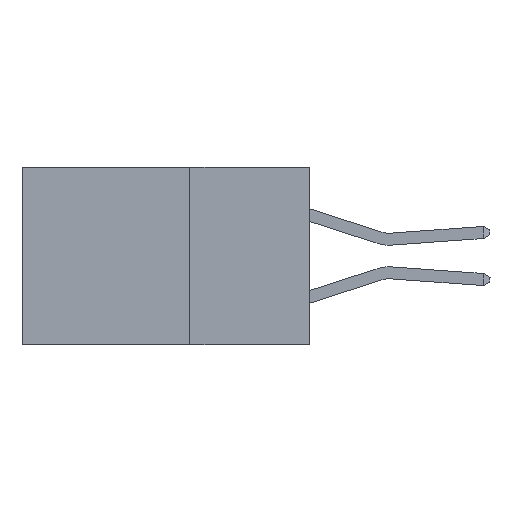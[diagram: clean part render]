
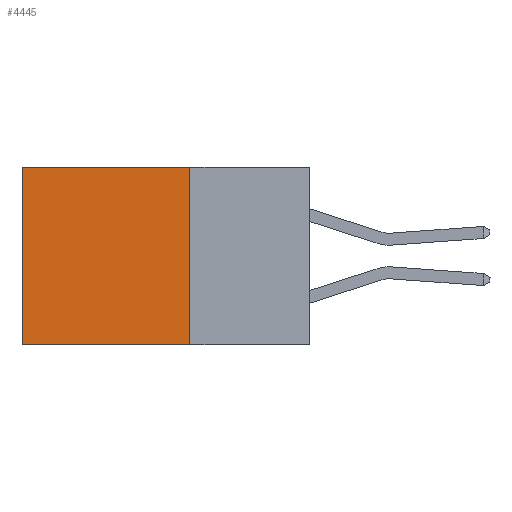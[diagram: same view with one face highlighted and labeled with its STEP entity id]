
A CAD part, left-side view. The second image highlights one B-rep face of the part: STEP entity #4445.
In plain terms, the highlighted planar face has unit normal (-1, 0, 0).
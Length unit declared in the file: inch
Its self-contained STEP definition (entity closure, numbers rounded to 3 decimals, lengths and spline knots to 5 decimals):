
#317 = EDGE_CURVE ( 'NONE', #3598, #5540, #5479, .T. ) ;
#974 = ORIENTED_EDGE ( 'NONE', *, *, #4265, .F. ) ;
#1936 = DIRECTION ( 'NONE',  ( 0., 0., -1. ) ) ;
#2107 = VECTOR ( 'NONE', #5605, 39.37008 ) ;
#2626 = EDGE_LOOP ( 'NONE', ( #6995, #974, #3247, #8632 ) ) ;
#2627 = LINE ( 'NONE', #6572, #8581 ) ;
#2744 = EDGE_CURVE ( 'NONE', #3598, #6791, #6237, .T. ) ;
#2918 = CARTESIAN_POINT ( 'NONE',  ( 0.298, 0.25, -0.37 ) ) ;
#3144 = LINE ( 'NONE', #2918, #8501 ) ;
#3247 = ORIENTED_EDGE ( 'NONE', *, *, #317, .F. ) ;
#3266 = CARTESIAN_POINT ( 'NONE',  ( 0.298, 0.6, 0. ) ) ;
#3598 = VERTEX_POINT ( 'NONE', #4420 ) ;
#3642 = FACE_OUTER_BOUND ( 'NONE', #2626, .T. ) ;
#3673 = DIRECTION ( 'NONE',  ( 0., 1., 0. ) ) ;
#4136 = CARTESIAN_POINT ( 'NONE',  ( 0.298, 0.25, 0. ) ) ;
#4265 = EDGE_CURVE ( 'NONE', #5540, #5332, #3144, .T. ) ;
#4420 = CARTESIAN_POINT ( 'NONE',  ( 0.298, 0.25, 0. ) ) ;
#4445 = ADVANCED_FACE ( 'NONE', ( #3642 ), #5028, .F. ) ;
#5028 = PLANE ( 'NONE',  #7657 ) ;
#5332 = VERTEX_POINT ( 'NONE', #6177 ) ;
#5479 = LINE ( 'NONE', #9676, #9493 ) ;
#5540 = VERTEX_POINT ( 'NONE', #6692 ) ;
#5605 = DIRECTION ( 'NONE',  ( 0., 1., 0. ) ) ;
#6177 = CARTESIAN_POINT ( 'NONE',  ( 0.298, 0.6, -0.37 ) ) ;
#6237 = LINE ( 'NONE', #9410, #2107 ) ;
#6572 = CARTESIAN_POINT ( 'NONE',  ( 0.298, 0.6, 0. ) ) ;
#6657 = EDGE_CURVE ( 'NONE', #6791, #5332, #2627, .T. ) ;
#6679 = DIRECTION ( 'NONE',  ( 0., 0., -1. ) ) ;
#6692 = CARTESIAN_POINT ( 'NONE',  ( 0.298, 0.25, -0.37 ) ) ;
#6791 = VERTEX_POINT ( 'NONE', #3266 ) ;
#6995 = ORIENTED_EDGE ( 'NONE', *, *, #6657, .T. ) ;
#7657 = AXIS2_PLACEMENT_3D ( 'NONE', #4136, #9627, #1936 ) ;
#8501 = VECTOR ( 'NONE', #3673, 39.37008 ) ;
#8581 = VECTOR ( 'NONE', #6679, 39.37008 ) ;
#8632 = ORIENTED_EDGE ( 'NONE', *, *, #2744, .T. ) ;
#8844 = DIRECTION ( 'NONE',  ( 0., 0., -1. ) ) ;
#9410 = CARTESIAN_POINT ( 'NONE',  ( 0.298, 0.25, 0. ) ) ;
#9493 = VECTOR ( 'NONE', #8844, 39.37008 ) ;
#9627 = DIRECTION ( 'NONE',  ( 1., 0., 0. ) ) ;
#9676 = CARTESIAN_POINT ( 'NONE',  ( 0.298, 0.25, 0. ) ) ;
